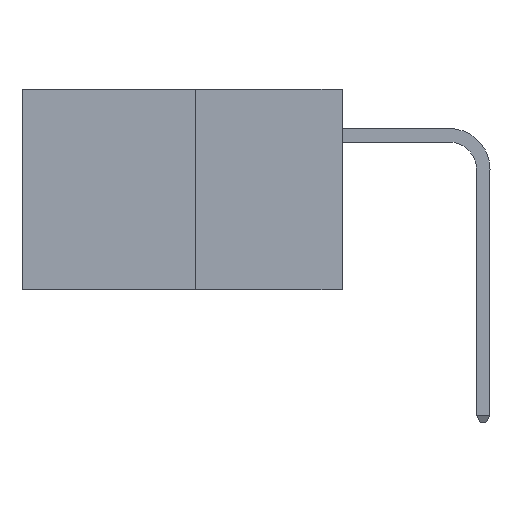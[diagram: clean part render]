
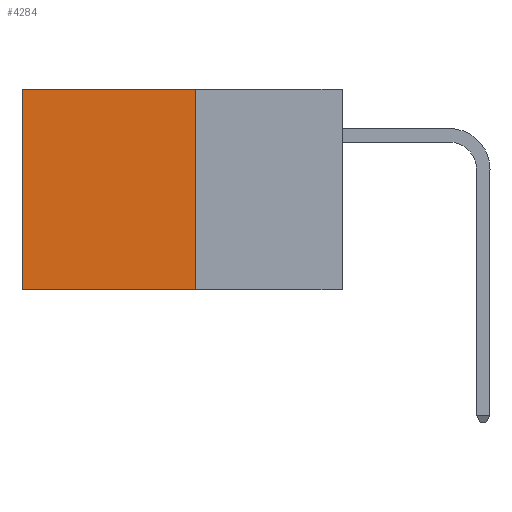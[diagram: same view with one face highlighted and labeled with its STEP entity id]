
A CAD part, left-side view. The second image highlights one B-rep face of the part: STEP entity #4284.
In plain terms, the highlighted planar face has unit normal (-1, 0, 0).
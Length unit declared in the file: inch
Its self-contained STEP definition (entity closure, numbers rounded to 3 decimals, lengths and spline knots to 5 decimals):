
#261 = CARTESIAN_POINT ( 'NONE',  ( 0.277, 0.27, -0.37 ) ) ;
#492 = LINE ( 'NONE', #5955, #5569 ) ;
#732 = ORIENTED_EDGE ( 'NONE', *, *, #6006, .T. ) ;
#1081 = VECTOR ( 'NONE', #1289, 39.37008 ) ;
#1289 = DIRECTION ( 'NONE',  ( 0., 0., -1. ) ) ;
#1889 = ORIENTED_EDGE ( 'NONE', *, *, #11941, .F. ) ;
#3002 = VERTEX_POINT ( 'NONE', #28856 ) ;
#3808 = CARTESIAN_POINT ( 'NONE',  ( 0.277, 0.27, 0. ) ) ;
#4284 = ADVANCED_FACE ( 'NONE', ( #24338 ), #6326, .F. ) ;
#5034 = CARTESIAN_POINT ( 'NONE',  ( 0.277, 0.27, -0.37 ) ) ;
#5569 = VECTOR ( 'NONE', #18295, 39.37008 ) ;
#5955 = CARTESIAN_POINT ( 'NONE',  ( 0.277, 0.27, 0. ) ) ;
#6006 = EDGE_CURVE ( 'NONE', #3002, #19511, #16854, .T. ) ;
#6326 = PLANE ( 'NONE',  #30965 ) ;
#7211 = LINE ( 'NONE', #5034, #27724 ) ;
#7720 = LINE ( 'NONE', #28510, #1081 ) ;
#8804 = DIRECTION ( 'NONE',  ( 0., 0., -1. ) ) ;
#8967 = CARTESIAN_POINT ( 'NONE',  ( 0.277, 0.59, -0.37 ) ) ;
#9489 = VECTOR ( 'NONE', #27883, 39.37008 ) ;
#11941 = EDGE_CURVE ( 'NONE', #16867, #19511, #7211, .T. ) ;
#16612 = ORIENTED_EDGE ( 'NONE', *, *, #20829, .F. ) ;
#16646 = ORIENTED_EDGE ( 'NONE', *, *, #23575, .T. ) ;
#16854 = LINE ( 'NONE', #17933, #9489 ) ;
#16867 = VERTEX_POINT ( 'NONE', #261 ) ;
#17933 = CARTESIAN_POINT ( 'NONE',  ( 0.277, 0.59, -0.37 ) ) ;
#18295 = DIRECTION ( 'NONE',  ( 0., 1., 0. ) ) ;
#18670 = CARTESIAN_POINT ( 'NONE',  ( 0.277, 0.27, -0.37 ) ) ;
#19379 = EDGE_LOOP ( 'NONE', ( #732, #1889, #16612, #16646 ) ) ;
#19511 = VERTEX_POINT ( 'NONE', #8967 ) ;
#20829 = EDGE_CURVE ( 'NONE', #20841, #16867, #7720, .T. ) ;
#20841 = VERTEX_POINT ( 'NONE', #3808 ) ;
#22356 = DIRECTION ( 'NONE',  ( 0., 1., 0. ) ) ;
#23575 = EDGE_CURVE ( 'NONE', #20841, #3002, #492, .T. ) ;
#23642 = DIRECTION ( 'NONE',  ( 1., 0., 0. ) ) ;
#24338 = FACE_OUTER_BOUND ( 'NONE', #19379, .T. ) ;
#27724 = VECTOR ( 'NONE', #22356, 39.37008 ) ;
#27883 = DIRECTION ( 'NONE',  ( 0., 0., -1. ) ) ;
#28510 = CARTESIAN_POINT ( 'NONE',  ( 0.277, 0.27, -0.37 ) ) ;
#28856 = CARTESIAN_POINT ( 'NONE',  ( 0.277, 0.59, 0. ) ) ;
#30965 = AXIS2_PLACEMENT_3D ( 'NONE', #18670, #23642, #8804 ) ;
